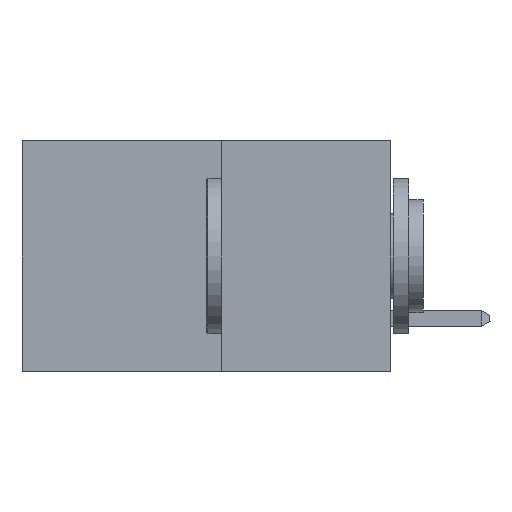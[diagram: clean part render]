
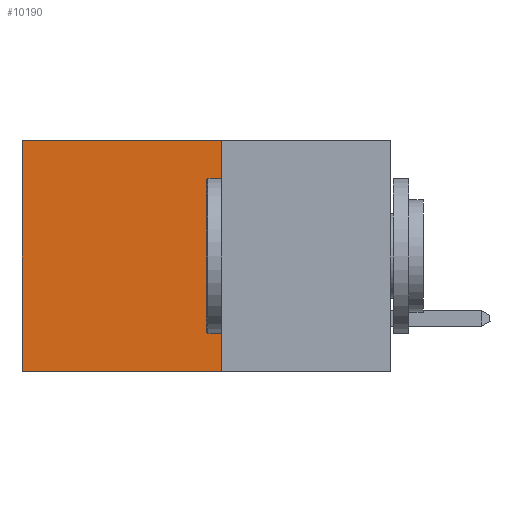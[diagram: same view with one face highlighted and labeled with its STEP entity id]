
A CAD part, left-side view. The second image highlights one B-rep face of the part: STEP entity #10190.
In plain terms, the highlighted planar face has unit normal (-1, 0, 0).
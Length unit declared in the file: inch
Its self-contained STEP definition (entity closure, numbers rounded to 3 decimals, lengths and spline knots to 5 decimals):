
#1670 = EDGE_LOOP ( 'NONE', ( #13283, #21849, #3067, #11000 ) ) ;
#2167 = CARTESIAN_POINT ( 'NONE',  ( 0.277, 0.27, -0.37 ) ) ;
#2604 = DIRECTION ( 'NONE',  ( 0., 1., 0. ) ) ;
#2683 = EDGE_CURVE ( 'NONE', #27175, #18777, #26469, .T. ) ;
#3067 = ORIENTED_EDGE ( 'NONE', *, *, #21335, .F. ) ;
#3252 = LINE ( 'NONE', #19775, #9862 ) ;
#4672 = DIRECTION ( 'NONE',  ( 1., 0., 0. ) ) ;
#6285 = CARTESIAN_POINT ( 'NONE',  ( 0.277, 0.27, -0.37 ) ) ;
#6879 = EDGE_CURVE ( 'NONE', #17012, #18777, #17460, .T. ) ;
#7787 = VECTOR ( 'NONE', #13853, 39.37008 ) ;
#8615 = CARTESIAN_POINT ( 'NONE',  ( 0.277, 0.59, -0.37 ) ) ;
#9862 = VECTOR ( 'NONE', #2604, 39.37008 ) ;
#10190 = ADVANCED_FACE ( 'NONE', ( #11856 ), #16890, .F. ) ;
#11000 = ORIENTED_EDGE ( 'NONE', *, *, #12404, .T. ) ;
#11400 = CARTESIAN_POINT ( 'NONE',  ( 0.277, 0.27, -0.37 ) ) ;
#11795 = CARTESIAN_POINT ( 'NONE',  ( 0.277, 0.27, 0. ) ) ;
#11856 = FACE_OUTER_BOUND ( 'NONE', #1670, .T. ) ;
#11974 = DIRECTION ( 'NONE',  ( 0., 1., 0. ) ) ;
#12404 = EDGE_CURVE ( 'NONE', #20824, #27175, #3252, .T. ) ;
#12546 = VECTOR ( 'NONE', #25801, 39.37008 ) ;
#12681 = CARTESIAN_POINT ( 'NONE',  ( 0.277, 0.27, -0.37 ) ) ;
#13283 = ORIENTED_EDGE ( 'NONE', *, *, #2683, .T. ) ;
#13853 = DIRECTION ( 'NONE',  ( 0., 0., -1. ) ) ;
#16890 = PLANE ( 'NONE',  #23980 ) ;
#17012 = VERTEX_POINT ( 'NONE', #11400 ) ;
#17460 = LINE ( 'NONE', #12681, #30243 ) ;
#18288 = LINE ( 'NONE', #6285, #12546 ) ;
#18777 = VERTEX_POINT ( 'NONE', #8615 ) ;
#19775 = CARTESIAN_POINT ( 'NONE',  ( 0.277, 0.27, 0. ) ) ;
#20667 = CARTESIAN_POINT ( 'NONE',  ( 0.277, 0.59, -0.37 ) ) ;
#20824 = VERTEX_POINT ( 'NONE', #11795 ) ;
#21335 = EDGE_CURVE ( 'NONE', #20824, #17012, #18288, .T. ) ;
#21809 = DIRECTION ( 'NONE',  ( 0., 0., -1. ) ) ;
#21849 = ORIENTED_EDGE ( 'NONE', *, *, #6879, .F. ) ;
#23980 = AXIS2_PLACEMENT_3D ( 'NONE', #2167, #4672, #21809 ) ;
#25801 = DIRECTION ( 'NONE',  ( 0., 0., -1. ) ) ;
#26469 = LINE ( 'NONE', #20667, #7787 ) ;
#27175 = VERTEX_POINT ( 'NONE', #29125 ) ;
#29125 = CARTESIAN_POINT ( 'NONE',  ( 0.277, 0.59, 0. ) ) ;
#30243 = VECTOR ( 'NONE', #11974, 39.37008 ) ;
